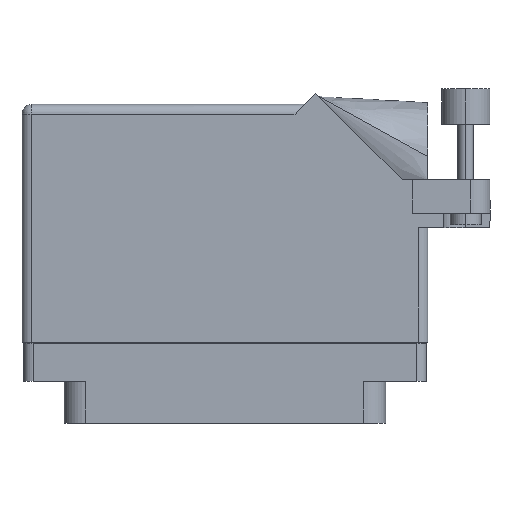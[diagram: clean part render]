
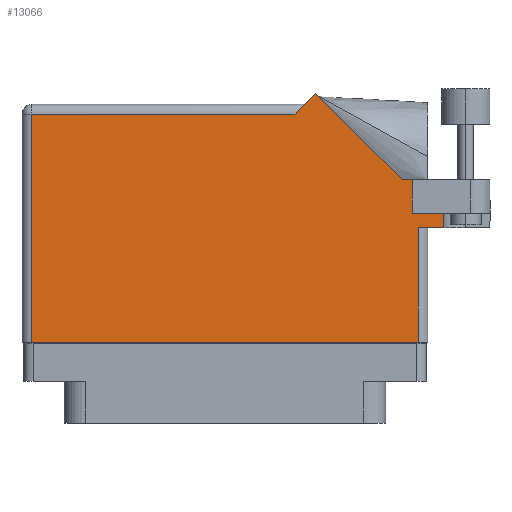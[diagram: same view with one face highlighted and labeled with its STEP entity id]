
A CAD part, front view. The second image highlights one B-rep face of the part: STEP entity #13066.
In plain terms, the highlighted face is planar.
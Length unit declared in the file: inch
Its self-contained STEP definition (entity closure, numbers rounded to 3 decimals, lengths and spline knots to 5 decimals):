
#149 = VECTOR ( 'NONE', #11543, 39.37008 ) ;
#802 = VECTOR ( 'NONE', #20610, 39.37008 ) ;
#867 = CARTESIAN_POINT ( 'NONE',  ( 1.206, 0.731, 0.455 ) ) ;
#1331 = VERTEX_POINT ( 'NONE', #24905 ) ;
#2341 = DIRECTION ( 'NONE',  ( 1., 0., 0. ) ) ;
#2722 = DIRECTION ( 'NONE',  ( -0.707, 0.707, 0. ) ) ;
#2775 = PLANE ( 'NONE',  #38021 ) ;
#3266 = LINE ( 'NONE', #35699, #22116 ) ;
#3991 = LINE ( 'NONE', #26176, #5204 ) ;
#5204 = VECTOR ( 'NONE', #33430, 39.37008 ) ;
#5663 = ORIENTED_EDGE ( 'NONE', *, *, #49081, .T. ) ;
#6450 = LINE ( 'NONE', #36400, #149 ) ;
#6534 = VECTOR ( 'NONE', #2341, 39.37008 ) ;
#7128 = LINE ( 'NONE', #28581, #802 ) ;
#7276 = VECTOR ( 'NONE', #16772, 39.37008 ) ;
#8434 = EDGE_CURVE ( 'NONE', #20907, #41438, #6450, .T. ) ;
#9008 = ORIENTED_EDGE ( 'NONE', *, *, #48699, .T. ) ;
#9397 = CARTESIAN_POINT ( 'NONE',  ( -1.306, -0.1, 0.455 ) ) ;
#9951 = ORIENTED_EDGE ( 'NONE', *, *, #20979, .F. ) ;
#10566 = ORIENTED_EDGE ( 'NONE', *, *, #35581, .T. ) ;
#10855 = DIRECTION ( 'NONE',  ( -1., 0., 0. ) ) ;
#11543 = DIRECTION ( 'NONE',  ( -1., 0., 0. ) ) ;
#11578 = ORIENTED_EDGE ( 'NONE', *, *, #35508, .F. ) ;
#13041 = CARTESIAN_POINT ( 'NONE',  ( 1.4075, 1.06177, 0.455 ) ) ;
#13066 = ADVANCED_FACE ( 'NONE', ( #35151 ), #2775, .F. ) ;
#13667 = VERTEX_POINT ( 'NONE', #31055 ) ;
#14169 = VECTOR ( 'NONE', #2722, 39.37008 ) ;
#14391 = DIRECTION ( 'NONE',  ( 0., 1., 0. ) ) ;
#14967 = EDGE_CURVE ( 'NONE', #32796, #13667, #3266, .T. ) ;
#15012 = CARTESIAN_POINT ( 'NONE',  ( 1.14042, 0.944, 0.455 ) ) ;
#15900 = CARTESIAN_POINT ( 'NONE',  ( 0.58371, 1.50071, 0.455 ) ) ;
#16772 = DIRECTION ( 'NONE',  ( 1., 0., 0. ) ) ;
#20610 = DIRECTION ( 'NONE',  ( 0., -1., 0. ) ) ;
#20907 = VERTEX_POINT ( 'NONE', #40891 ) ;
#20979 = EDGE_CURVE ( 'NONE', #52148, #42815, #3991, .T. ) ;
#21004 = VERTEX_POINT ( 'NONE', #29540 ) ;
#21028 = LINE ( 'NONE', #9397, #6534 ) ;
#21465 = DIRECTION ( 'NONE',  ( 0., -1., 0. ) ) ;
#21513 = CARTESIAN_POINT ( 'NONE',  ( 1.306, 0.637, 0.455 ) ) ;
#21564 = CARTESIAN_POINT ( 'NONE',  ( 1.206, 0.731, 0.455 ) ) ;
#21735 = EDGE_LOOP ( 'NONE', ( #9008, #47676, #36672, #11578, #9951, #51082, #51873, #43397, #43464, #10566, #5663 ) ) ;
#22116 = VECTOR ( 'NONE', #27971, 39.37008 ) ;
#24019 = CARTESIAN_POINT ( 'NONE',  ( 1.244, 0.637, 0.455 ) ) ;
#24582 = LINE ( 'NONE', #13041, #39737 ) ;
#24905 = CARTESIAN_POINT ( 'NONE',  ( 1.4075, 0.637, 0.455 ) ) ;
#24990 = EDGE_CURVE ( 'NONE', #42712, #1331, #50798, .T. ) ;
#25345 = CARTESIAN_POINT ( 'NONE',  ( 1.4075, 0.731, 0.455 ) ) ;
#26060 = DIRECTION ( 'NONE',  ( -1., 0., 0. ) ) ;
#26176 = CARTESIAN_POINT ( 'NONE',  ( 1.206, 0.731, 0.455 ) ) ;
#26549 = CARTESIAN_POINT ( 'NONE',  ( 1.244, 0.637, 0.455 ) ) ;
#27971 = DIRECTION ( 'NONE',  ( -0.707, -0.707, 0. ) ) ;
#28581 = CARTESIAN_POINT ( 'NONE',  ( -1.244, -0.1, 0.455 ) ) ;
#28920 = DIRECTION ( 'NONE',  ( 0., 1., 0. ) ) ;
#28982 = EDGE_CURVE ( 'NONE', #45098, #42712, #30818, .T. ) ;
#29540 = CARTESIAN_POINT ( 'NONE',  ( -1.244, 1.368, 0.455 ) ) ;
#30818 = LINE ( 'NONE', #26549, #51027 ) ;
#30947 = CARTESIAN_POINT ( 'NONE',  ( -1.306, 1.43, 0.455 ) ) ;
#31055 = CARTESIAN_POINT ( 'NONE',  ( 0.451, 1.368, 0.455 ) ) ;
#32053 = VECTOR ( 'NONE', #28920, 39.37008 ) ;
#32491 = LINE ( 'NONE', #15012, #14169 ) ;
#32796 = VERTEX_POINT ( 'NONE', #15900 ) ;
#33430 = DIRECTION ( 'NONE',  ( 1., 0., 0. ) ) ;
#35002 = DIRECTION ( 'NONE',  ( 0., 0., -1. ) ) ;
#35151 = FACE_OUTER_BOUND ( 'NONE', #21735, .T. ) ;
#35508 = EDGE_CURVE ( 'NONE', #42815, #1331, #24582, .T. ) ;
#35581 = EDGE_CURVE ( 'NONE', #13667, #21004, #47885, .T. ) ;
#35699 = CARTESIAN_POINT ( 'NONE',  ( 0.513, 1.43, 0.455 ) ) ;
#36400 = CARTESIAN_POINT ( 'NONE',  ( 1.706, 0.944, 0.455 ) ) ;
#36672 = ORIENTED_EDGE ( 'NONE', *, *, #24990, .T. ) ;
#38021 = AXIS2_PLACEMENT_3D ( 'NONE', #30947, #35002, #10855 ) ;
#38099 = CARTESIAN_POINT ( 'NONE',  ( 1.14042, 0.944, 0.455 ) ) ;
#38117 = EDGE_CURVE ( 'NONE', #41438, #32796, #32491, .T. ) ;
#39528 = CARTESIAN_POINT ( 'NONE',  ( -1.244, -0.1, 0.455 ) ) ;
#39737 = VECTOR ( 'NONE', #21465, 39.37008 ) ;
#40891 = CARTESIAN_POINT ( 'NONE',  ( 1.206, 0.944, 0.455 ) ) ;
#41438 = VERTEX_POINT ( 'NONE', #38099 ) ;
#41915 = EDGE_CURVE ( 'NONE', #52148, #20907, #45283, .T. ) ;
#42712 = VERTEX_POINT ( 'NONE', #24019 ) ;
#42815 = VERTEX_POINT ( 'NONE', #25345 ) ;
#43397 = ORIENTED_EDGE ( 'NONE', *, *, #38117, .T. ) ;
#43464 = ORIENTED_EDGE ( 'NONE', *, *, #14967, .T. ) ;
#45098 = VERTEX_POINT ( 'NONE', #47875 ) ;
#45283 = LINE ( 'NONE', #867, #32053 ) ;
#45873 = VERTEX_POINT ( 'NONE', #39528 ) ;
#46317 = CARTESIAN_POINT ( 'NONE',  ( -1.306, 1.368, 0.455 ) ) ;
#47676 = ORIENTED_EDGE ( 'NONE', *, *, #28982, .T. ) ;
#47875 = CARTESIAN_POINT ( 'NONE',  ( 1.244, -0.1, 0.455 ) ) ;
#47885 = LINE ( 'NONE', #46317, #49148 ) ;
#48699 = EDGE_CURVE ( 'NONE', #45873, #45098, #21028, .T. ) ;
#49081 = EDGE_CURVE ( 'NONE', #21004, #45873, #7128, .T. ) ;
#49148 = VECTOR ( 'NONE', #26060, 39.37008 ) ;
#50798 = LINE ( 'NONE', #21513, #7276 ) ;
#51027 = VECTOR ( 'NONE', #14391, 39.37008 ) ;
#51082 = ORIENTED_EDGE ( 'NONE', *, *, #41915, .T. ) ;
#51873 = ORIENTED_EDGE ( 'NONE', *, *, #8434, .T. ) ;
#52148 = VERTEX_POINT ( 'NONE', #21564 ) ;
